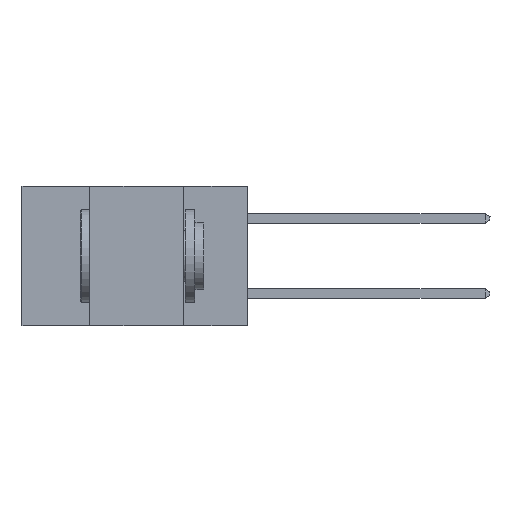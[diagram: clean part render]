
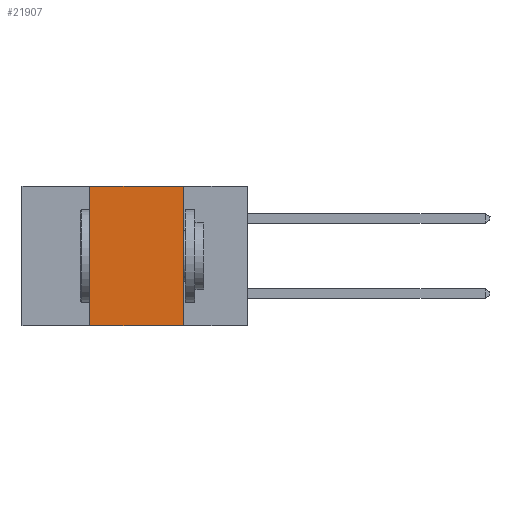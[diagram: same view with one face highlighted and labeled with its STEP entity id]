
A CAD part, left-side view. The second image highlights one B-rep face of the part: STEP entity #21907.
In plain terms, the highlighted planar face has unit normal (-1, 0, 0).
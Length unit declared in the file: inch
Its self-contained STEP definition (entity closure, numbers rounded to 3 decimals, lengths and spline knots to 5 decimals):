
#312 = ORIENTED_EDGE ( 'NONE', *, *, #8101, .T. ) ;
#632 = DIRECTION ( 'NONE',  ( 1., 0., 0. ) ) ;
#1060 = CARTESIAN_POINT ( 'NONE',  ( 0., 0.42, 0. ) ) ;
#1455 = DIRECTION ( 'NONE',  ( 0., -1., 0. ) ) ;
#2818 = PLANE ( 'NONE',  #22275 ) ;
#3306 = CARTESIAN_POINT ( 'NONE',  ( 0., 0.42, -0.37 ) ) ;
#4539 = FACE_OUTER_BOUND ( 'NONE', #8103, .T. ) ;
#4631 = CARTESIAN_POINT ( 'NONE',  ( 0., 0.17, -0.37 ) ) ;
#4773 = EDGE_CURVE ( 'NONE', #18350, #21495, #10190, .T. ) ;
#5359 = EDGE_CURVE ( 'NONE', #6587, #18350, #18279, .T. ) ;
#5663 = VECTOR ( 'NONE', #16334, 39.37008 ) ;
#6149 = CARTESIAN_POINT ( 'NONE',  ( 0., 0.17, -0.37 ) ) ;
#6587 = VERTEX_POINT ( 'NONE', #3306 ) ;
#6663 = LINE ( 'NONE', #4631, #9067 ) ;
#6847 = VECTOR ( 'NONE', #7080, 39.37008 ) ;
#6872 = ORIENTED_EDGE ( 'NONE', *, *, #22625, .F. ) ;
#7080 = DIRECTION ( 'NONE',  ( 0., -1., 0. ) ) ;
#7500 = ORIENTED_EDGE ( 'NONE', *, *, #4773, .F. ) ;
#8101 = EDGE_CURVE ( 'NONE', #6587, #21887, #12141, .T. ) ;
#8103 = EDGE_LOOP ( 'NONE', ( #6872, #7500, #9578, #312 ) ) ;
#8993 = VECTOR ( 'NONE', #1455, 39.37008 ) ;
#9067 = VECTOR ( 'NONE', #11622, 39.37008 ) ;
#9578 = ORIENTED_EDGE ( 'NONE', *, *, #5359, .F. ) ;
#10190 = LINE ( 'NONE', #17191, #8993 ) ;
#10414 = CARTESIAN_POINT ( 'NONE',  ( 0., 0.6, -0.37 ) ) ;
#11199 = CARTESIAN_POINT ( 'NONE',  ( 0., 0.6, 0. ) ) ;
#11622 = DIRECTION ( 'NONE',  ( 0., 0., -1. ) ) ;
#12141 = LINE ( 'NONE', #10414, #6847 ) ;
#12659 = CARTESIAN_POINT ( 'NONE',  ( 0., 0.42, -0.37 ) ) ;
#16334 = DIRECTION ( 'NONE',  ( 0., 0., 1. ) ) ;
#16374 = DIRECTION ( 'NONE',  ( 0., 0., -1. ) ) ;
#17191 = CARTESIAN_POINT ( 'NONE',  ( 0., 0.6, 0. ) ) ;
#18279 = LINE ( 'NONE', #12659, #5663 ) ;
#18350 = VERTEX_POINT ( 'NONE', #1060 ) ;
#20397 = CARTESIAN_POINT ( 'NONE',  ( 0., 0.17, 0. ) ) ;
#21495 = VERTEX_POINT ( 'NONE', #20397 ) ;
#21887 = VERTEX_POINT ( 'NONE', #6149 ) ;
#21907 = ADVANCED_FACE ( 'NONE', ( #4539 ), #2818, .F. ) ;
#22275 = AXIS2_PLACEMENT_3D ( 'NONE', #11199, #632, #16374 ) ;
#22625 = EDGE_CURVE ( 'NONE', #21495, #21887, #6663, .T. ) ;
